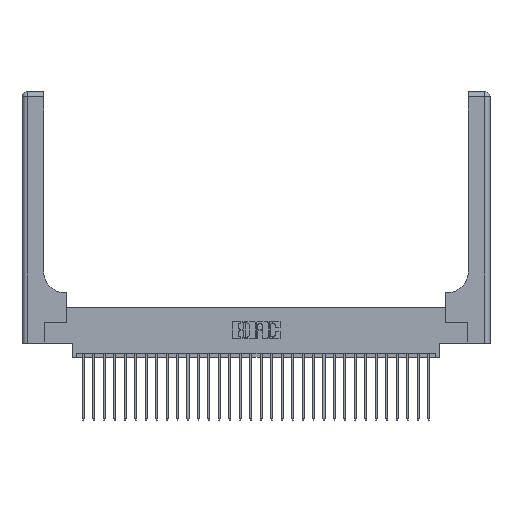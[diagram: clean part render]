
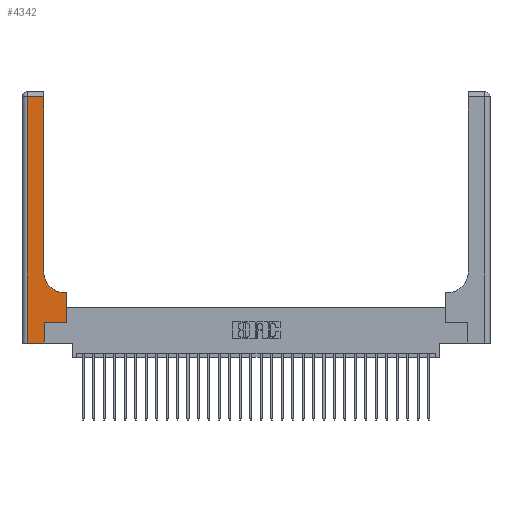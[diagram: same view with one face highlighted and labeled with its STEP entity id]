
A CAD part, top view. The second image highlights one B-rep face of the part: STEP entity #4342.
In plain terms, the highlighted planar face has unit normal (0, 0, 1).
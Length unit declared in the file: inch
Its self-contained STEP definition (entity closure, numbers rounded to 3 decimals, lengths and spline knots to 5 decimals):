
#431 = VERTEX_POINT ( 'NONE', #14664 ) ;
#857 = VERTEX_POINT ( 'NONE', #1756 ) ;
#1087 = DIRECTION ( 'NONE',  ( 1., 0., 0. ) ) ;
#1221 = LINE ( 'NONE', #1364, #11200 ) ;
#1238 = DIRECTION ( 'NONE',  ( 1., 0., 0. ) ) ;
#1364 = CARTESIAN_POINT ( 'NONE',  ( 0.26, 3., 0.37 ) ) ;
#1756 = CARTESIAN_POINT ( 'NONE',  ( 0.26, 0.85, 0.37 ) ) ;
#2277 = CARTESIAN_POINT ( 'NONE',  ( 0.528, 0.25, 0.37 ) ) ;
#2461 = AXIS2_PLACEMENT_3D ( 'NONE', #14637, #23591, #9275 ) ;
#2550 = VECTOR ( 'NONE', #4468, 39.37008 ) ;
#2897 = EDGE_CURVE ( 'NONE', #16435, #18538, #6084, .T. ) ;
#3586 = DIRECTION ( 'NONE',  ( 0., 1., 0. ) ) ;
#4031 = EDGE_CURVE ( 'NONE', #26582, #431, #13314, .T. ) ;
#4178 = LINE ( 'NONE', #15509, #8767 ) ;
#4342 = ADVANCED_FACE ( 'NONE', ( #23454 ), #7846, .F. ) ;
#4468 = DIRECTION ( 'NONE',  ( 1., 0., 0. ) ) ;
#4729 = ORIENTED_EDGE ( 'NONE', *, *, #10106, .T. ) ;
#4778 = EDGE_CURVE ( 'NONE', #10034, #857, #20321, .T. ) ;
#5053 = VERTEX_POINT ( 'NONE', #11513 ) ;
#5515 = CARTESIAN_POINT ( 'NONE',  ( 0.265, 0., 0.37 ) ) ;
#5756 = ORIENTED_EDGE ( 'NONE', *, *, #13000, .T. ) ;
#6084 = LINE ( 'NONE', #24610, #2550 ) ;
#6504 = DIRECTION ( 'NONE',  ( 0., -1., 0. ) ) ;
#7846 = PLANE ( 'NONE',  #2461 ) ;
#7919 = ORIENTED_EDGE ( 'NONE', *, *, #2897, .T. ) ;
#8767 = VECTOR ( 'NONE', #6504, 39.37008 ) ;
#9271 = VECTOR ( 'NONE', #1238, 39.37008 ) ;
#9275 = DIRECTION ( 'NONE',  ( -1., 0., 0. ) ) ;
#9679 = CARTESIAN_POINT ( 'NONE',  ( 0.06, 0., 0.37 ) ) ;
#9959 = ORIENTED_EDGE ( 'NONE', *, *, #4031, .T. ) ;
#10034 = VERTEX_POINT ( 'NONE', #23021 ) ;
#10106 = EDGE_CURVE ( 'NONE', #431, #10034, #11987, .T. ) ;
#10120 = EDGE_LOOP ( 'NONE', ( #19116, #5756, #16038, #7919, #23682, #27086, #9959, #4729, #26859 ) ) ;
#10287 = CARTESIAN_POINT ( 'NONE',  ( 0., 2.94, 0.37 ) ) ;
#11200 = VECTOR ( 'NONE', #3586, 39.37008 ) ;
#11255 = DIRECTION ( 'NONE',  ( 0., 1., 0. ) ) ;
#11513 = CARTESIAN_POINT ( 'NONE',  ( 0.06, 2.94, 0.37 ) ) ;
#11987 = LINE ( 'NONE', #14502, #25534 ) ;
#13000 = EDGE_CURVE ( 'NONE', #25521, #5053, #25577, .T. ) ;
#13314 = LINE ( 'NONE', #2277, #26070 ) ;
#13886 = EDGE_CURVE ( 'NONE', #18538, #28933, #25654, .T. ) ;
#14502 = CARTESIAN_POINT ( 'NONE',  ( 0.26, 0.6, 0.37 ) ) ;
#14637 = CARTESIAN_POINT ( 'NONE',  ( 0., 3., 0.37 ) ) ;
#14664 = CARTESIAN_POINT ( 'NONE',  ( 0.528, 0.6, 0.37 ) ) ;
#15127 = EDGE_CURVE ( 'NONE', #28933, #26582, #23475, .T. ) ;
#15337 = CARTESIAN_POINT ( 'NONE',  ( 0.265, 0.25, 0.37 ) ) ;
#15509 = CARTESIAN_POINT ( 'NONE',  ( 0.06, 3., 0.37 ) ) ;
#15654 = CARTESIAN_POINT ( 'NONE',  ( 0.26, 2.94, 0.37 ) ) ;
#15744 = VECTOR ( 'NONE', #19051, 39.37008 ) ;
#16038 = ORIENTED_EDGE ( 'NONE', *, *, #19240, .T. ) ;
#16435 = VERTEX_POINT ( 'NONE', #9679 ) ;
#16922 = DIRECTION ( 'NONE',  ( -1., 0., 0. ) ) ;
#18538 = VERTEX_POINT ( 'NONE', #22646 ) ;
#18560 = VECTOR ( 'NONE', #16922, 39.37008 ) ;
#19051 = DIRECTION ( 'NONE',  ( 0., 1., 0. ) ) ;
#19116 = ORIENTED_EDGE ( 'NONE', *, *, #20826, .T. ) ;
#19240 = EDGE_CURVE ( 'NONE', #5053, #16435, #4178, .T. ) ;
#19380 = CARTESIAN_POINT ( 'NONE',  ( 0.528, 0.25, 0.37 ) ) ;
#20321 = CIRCLE ( 'NONE', #28747, 0.25 ) ;
#20826 = EDGE_CURVE ( 'NONE', #857, #25521, #1221, .T. ) ;
#22646 = CARTESIAN_POINT ( 'NONE',  ( 0.265, 0., 0.37 ) ) ;
#22868 = DIRECTION ( 'NONE',  ( -1., 0., 0. ) ) ;
#23021 = CARTESIAN_POINT ( 'NONE',  ( 0.51, 0.6, 0.37 ) ) ;
#23041 = CARTESIAN_POINT ( 'NONE',  ( 0.265, 0.25, 0.37 ) ) ;
#23454 = FACE_OUTER_BOUND ( 'NONE', #10120, .T. ) ;
#23475 = LINE ( 'NONE', #23041, #9271 ) ;
#23591 = DIRECTION ( 'NONE',  ( 0., 0., -1. ) ) ;
#23682 = ORIENTED_EDGE ( 'NONE', *, *, #13886, .T. ) ;
#24610 = CARTESIAN_POINT ( 'NONE',  ( 0., 0., 0.37 ) ) ;
#25521 = VERTEX_POINT ( 'NONE', #15654 ) ;
#25534 = VECTOR ( 'NONE', #22868, 39.37008 ) ;
#25577 = LINE ( 'NONE', #10287, #18560 ) ;
#25646 = DIRECTION ( 'NONE',  ( 0., 0., -1. ) ) ;
#25654 = LINE ( 'NONE', #5515, #15744 ) ;
#26070 = VECTOR ( 'NONE', #11255, 39.37008 ) ;
#26582 = VERTEX_POINT ( 'NONE', #19380 ) ;
#26859 = ORIENTED_EDGE ( 'NONE', *, *, #4778, .T. ) ;
#27086 = ORIENTED_EDGE ( 'NONE', *, *, #15127, .T. ) ;
#27403 = CARTESIAN_POINT ( 'NONE',  ( 0.51, 0.85, 0.37 ) ) ;
#28747 = AXIS2_PLACEMENT_3D ( 'NONE', #27403, #25646, #1087 ) ;
#28933 = VERTEX_POINT ( 'NONE', #15337 ) ;
